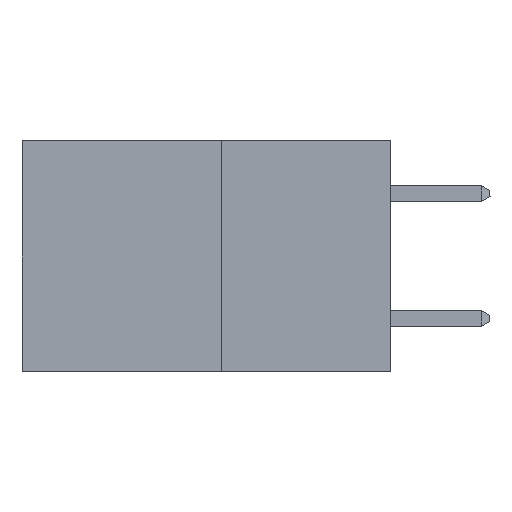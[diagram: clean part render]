
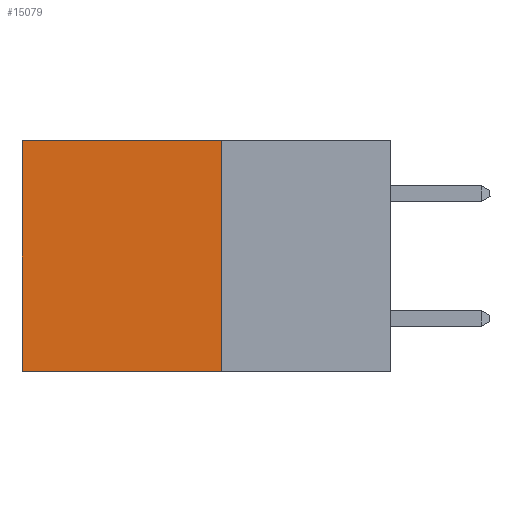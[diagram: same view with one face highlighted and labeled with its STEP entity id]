
A CAD part, left-side view. The second image highlights one B-rep face of the part: STEP entity #15079.
In plain terms, the highlighted planar face has unit normal (-1, 0, 0).
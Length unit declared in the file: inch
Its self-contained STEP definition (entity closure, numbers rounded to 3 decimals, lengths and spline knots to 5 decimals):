
#692 = FACE_OUTER_BOUND ( 'NONE', #23408, .T. ) ;
#826 = DIRECTION ( 'NONE',  ( 0., 0., -1. ) ) ;
#1962 = LINE ( 'NONE', #10953, #23740 ) ;
#3893 = LINE ( 'NONE', #34667, #11211 ) ;
#3909 = VERTEX_POINT ( 'NONE', #33902 ) ;
#4688 = VERTEX_POINT ( 'NONE', #17843 ) ;
#6285 = CARTESIAN_POINT ( 'NONE',  ( 0.277, 0.59, -0.37 ) ) ;
#7321 = CARTESIAN_POINT ( 'NONE',  ( 0.277, 0.27, -0.37 ) ) ;
#8579 = EDGE_CURVE ( 'NONE', #24749, #4688, #1962, .T. ) ;
#9054 = VERTEX_POINT ( 'NONE', #16176 ) ;
#9151 = ORIENTED_EDGE ( 'NONE', *, *, #12564, .F. ) ;
#9625 = EDGE_CURVE ( 'NONE', #3909, #9054, #18236, .T. ) ;
#10953 = CARTESIAN_POINT ( 'NONE',  ( 0.277, 0.27, 0. ) ) ;
#11211 = VECTOR ( 'NONE', #26465, 39.37008 ) ;
#11867 = VECTOR ( 'NONE', #18166, 39.37008 ) ;
#12007 = ORIENTED_EDGE ( 'NONE', *, *, #18319, .T. ) ;
#12564 = EDGE_CURVE ( 'NONE', #24749, #3909, #3893, .T. ) ;
#14960 = CARTESIAN_POINT ( 'NONE',  ( 0.277, 0.27, 0. ) ) ;
#15079 = ADVANCED_FACE ( 'NONE', ( #692 ), #29487, .F. ) ;
#16176 = CARTESIAN_POINT ( 'NONE',  ( 0.277, 0.59, -0.37 ) ) ;
#17843 = CARTESIAN_POINT ( 'NONE',  ( 0.277, 0.59, 0. ) ) ;
#18166 = DIRECTION ( 'NONE',  ( 0., 1., 0. ) ) ;
#18236 = LINE ( 'NONE', #7321, #11867 ) ;
#18319 = EDGE_CURVE ( 'NONE', #4688, #9054, #20547, .T. ) ;
#18665 = DIRECTION ( 'NONE',  ( 0., 0., -1. ) ) ;
#20547 = LINE ( 'NONE', #6285, #25235 ) ;
#23408 = EDGE_LOOP ( 'NONE', ( #12007, #27998, #9151, #30075 ) ) ;
#23740 = VECTOR ( 'NONE', #29960, 39.37008 ) ;
#24749 = VERTEX_POINT ( 'NONE', #14960 ) ;
#25235 = VECTOR ( 'NONE', #826, 39.37008 ) ;
#26465 = DIRECTION ( 'NONE',  ( 0., 0., -1. ) ) ;
#27998 = ORIENTED_EDGE ( 'NONE', *, *, #9625, .F. ) ;
#29487 = PLANE ( 'NONE',  #34297 ) ;
#29960 = DIRECTION ( 'NONE',  ( 0., 1., 0. ) ) ;
#30075 = ORIENTED_EDGE ( 'NONE', *, *, #8579, .T. ) ;
#32200 = CARTESIAN_POINT ( 'NONE',  ( 0.277, 0.27, -0.37 ) ) ;
#33902 = CARTESIAN_POINT ( 'NONE',  ( 0.277, 0.27, -0.37 ) ) ;
#34297 = AXIS2_PLACEMENT_3D ( 'NONE', #32200, #34955, #18665 ) ;
#34667 = CARTESIAN_POINT ( 'NONE',  ( 0.277, 0.27, -0.37 ) ) ;
#34955 = DIRECTION ( 'NONE',  ( 1., 0., 0. ) ) ;
